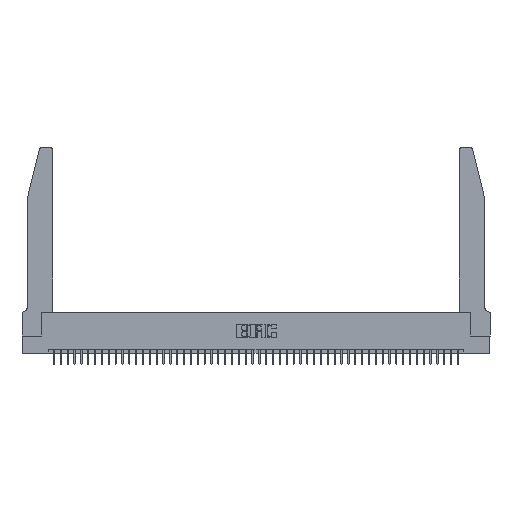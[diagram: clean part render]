
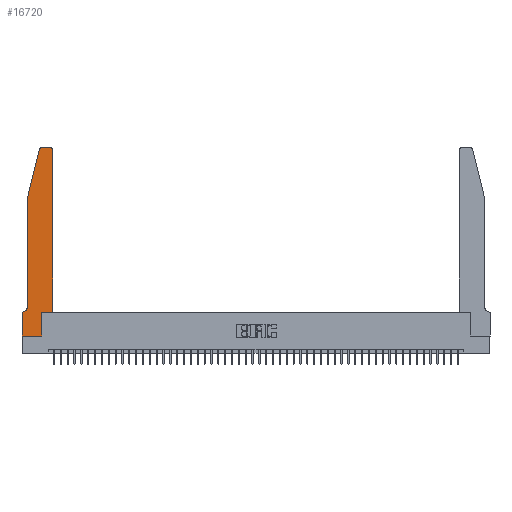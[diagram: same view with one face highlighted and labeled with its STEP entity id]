
A CAD part, top view. The second image highlights one B-rep face of the part: STEP entity #16720.
In plain terms, the highlighted planar face has unit normal (0, 0, 1).
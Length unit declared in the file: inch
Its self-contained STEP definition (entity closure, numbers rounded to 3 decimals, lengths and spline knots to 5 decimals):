
#959 = VERTEX_POINT ( 'NONE', #40195 ) ;
#1164 = DIRECTION ( 'NONE',  ( 0., -1., 0. ) ) ;
#1457 = VERTEX_POINT ( 'NONE', #7270 ) ;
#4528 = DIRECTION ( 'NONE',  ( 0., 0., 1. ) ) ;
#5020 = LINE ( 'NONE', #13585, #28966 ) ;
#5047 = VECTOR ( 'NONE', #10847, 39.37008 ) ;
#5134 = DIRECTION ( 'NONE',  ( 0., -1., 0. ) ) ;
#5814 = CARTESIAN_POINT ( 'NONE',  ( 0.4505, 0.35, 0.37 ) ) ;
#6054 = VERTEX_POINT ( 'NONE', #40809 ) ;
#6820 = CIRCLE ( 'NONE', #10229, 0.03 ) ;
#7005 = CARTESIAN_POINT ( 'NONE',  ( 0.4205, 2.72, 0.37 ) ) ;
#7157 = CARTESIAN_POINT ( 'NONE',  ( 0.0755, 2., 0.37 ) ) ;
#7270 = CARTESIAN_POINT ( 'NONE',  ( 0., 0.35, 0.37 ) ) ;
#7607 = CARTESIAN_POINT ( 'NONE',  ( 0.4205, 2.75, 0.37 ) ) ;
#8692 = CARTESIAN_POINT ( 'NONE',  ( 0.0755, 0.42, 0.37 ) ) ;
#9136 = EDGE_CURVE ( 'NONE', #26311, #43117, #32118, .T. ) ;
#9185 = VERTEX_POINT ( 'NONE', #48467 ) ;
#9391 = CARTESIAN_POINT ( 'NONE',  ( 0.4505, 2.72, 0.37 ) ) ;
#10101 = ORIENTED_EDGE ( 'NONE', *, *, #21083, .T. ) ;
#10229 = AXIS2_PLACEMENT_3D ( 'NONE', #7005, #22536, #26686 ) ;
#10551 = CARTESIAN_POINT ( 'NONE',  ( 0.2865, 0., 0.37 ) ) ;
#10623 = DIRECTION ( 'NONE',  ( 1., 0., 0. ) ) ;
#10847 = DIRECTION ( 'NONE',  ( -0.239, -0.971, 0. ) ) ;
#11303 = VERTEX_POINT ( 'NONE', #33861 ) ;
#11826 = VECTOR ( 'NONE', #21727, 39.37008 ) ;
#12398 = VECTOR ( 'NONE', #1164, 39.37008 ) ;
#12440 = DIRECTION ( 'NONE',  ( -1., 0., 0. ) ) ;
#12836 = ORIENTED_EDGE ( 'NONE', *, *, #31650, .T. ) ;
#13585 = CARTESIAN_POINT ( 'NONE',  ( 0.0755, 0.35, 0.37 ) ) ;
#13939 = CARTESIAN_POINT ( 'NONE',  ( 0., 0., 0.37 ) ) ;
#14050 = EDGE_CURVE ( 'NONE', #9185, #19016, #43178, .T. ) ;
#14434 = CARTESIAN_POINT ( 'NONE',  ( 0.4505, 0.35, 0.37 ) ) ;
#15198 = LINE ( 'NONE', #7157, #5047 ) ;
#15642 = DIRECTION ( 'NONE',  ( 1., 0., 0. ) ) ;
#15682 = VERTEX_POINT ( 'NONE', #44087 ) ;
#15969 = VERTEX_POINT ( 'NONE', #7607 ) ;
#16199 = PLANE ( 'NONE',  #27965 ) ;
#16534 = LINE ( 'NONE', #14434, #28512 ) ;
#16720 = ADVANCED_FACE ( 'NONE', ( #18972 ), #16199, .T. ) ;
#17407 = DIRECTION ( 'NONE',  ( -1., 0., 0. ) ) ;
#18972 = FACE_OUTER_BOUND ( 'NONE', #23552, .T. ) ;
#19016 = VERTEX_POINT ( 'NONE', #8692 ) ;
#19286 = ORIENTED_EDGE ( 'NONE', *, *, #9136, .T. ) ;
#19320 = ORIENTED_EDGE ( 'NONE', *, *, #38572, .T. ) ;
#21083 = EDGE_CURVE ( 'NONE', #41667, #15969, #6820, .T. ) ;
#21625 = VECTOR ( 'NONE', #39543, 39.37008 ) ;
#21727 = DIRECTION ( 'NONE',  ( 0., 1., 0. ) ) ;
#22536 = DIRECTION ( 'NONE',  ( 0., 0., 1. ) ) ;
#23552 = EDGE_LOOP ( 'NONE', ( #32612, #43770, #19320, #33153, #12836, #25225, #35252, #43160, #19286, #33865, #46588, #10101 ) ) ;
#24558 = CIRCLE ( 'NONE', #39953, 0.07 ) ;
#25225 = ORIENTED_EDGE ( 'NONE', *, *, #26791, .T. ) ;
#25535 = LINE ( 'NONE', #36167, #12398 ) ;
#26311 = VERTEX_POINT ( 'NONE', #10551 ) ;
#26686 = DIRECTION ( 'NONE',  ( 1., 0., 0. ) ) ;
#26791 = EDGE_CURVE ( 'NONE', #15682, #1457, #5020, .T. ) ;
#27951 = CARTESIAN_POINT ( 'NONE',  ( 0.0055, 0.42, 0.37 ) ) ;
#27965 = AXIS2_PLACEMENT_3D ( 'NONE', #38762, #4528, #35206 ) ;
#28012 = CARTESIAN_POINT ( 'NONE',  ( 0.0755, 2., 0.37 ) ) ;
#28512 = VECTOR ( 'NONE', #48211, 39.37008 ) ;
#28824 = LINE ( 'NONE', #5814, #21625 ) ;
#28966 = VECTOR ( 'NONE', #17407, 39.37008 ) ;
#30964 = CARTESIAN_POINT ( 'NONE',  ( 0.284, 2.72, 0.37 ) ) ;
#31107 = EDGE_CURVE ( 'NONE', #43117, #45739, #28824, .T. ) ;
#31618 = AXIS2_PLACEMENT_3D ( 'NONE', #30964, #35125, #15642 ) ;
#31650 = EDGE_CURVE ( 'NONE', #19016, #15682, #24558, .T. ) ;
#32118 = LINE ( 'NONE', #48303, #11826 ) ;
#32612 = ORIENTED_EDGE ( 'NONE', *, *, #36118, .T. ) ;
#32786 = EDGE_CURVE ( 'NONE', #11303, #6054, #47740, .T. ) ;
#33040 = LINE ( 'NONE', #34683, #37836 ) ;
#33153 = ORIENTED_EDGE ( 'NONE', *, *, #14050, .T. ) ;
#33861 = CARTESIAN_POINT ( 'NONE',  ( 0.284, 2.75, 0.37 ) ) ;
#33865 = ORIENTED_EDGE ( 'NONE', *, *, #31107, .T. ) ;
#34193 = DIRECTION ( 'NONE',  ( -1., 0., 0. ) ) ;
#34683 = CARTESIAN_POINT ( 'NONE',  ( 0.2605, 2.75, 0.37 ) ) ;
#35125 = DIRECTION ( 'NONE',  ( 0., 0., 1. ) ) ;
#35136 = VECTOR ( 'NONE', #10623, 39.37008 ) ;
#35206 = DIRECTION ( 'NONE',  ( 1., 0., 0. ) ) ;
#35252 = ORIENTED_EDGE ( 'NONE', *, *, #46805, .T. ) ;
#36118 = EDGE_CURVE ( 'NONE', #15969, #11303, #33040, .T. ) ;
#36167 = CARTESIAN_POINT ( 'NONE',  ( 0., 0., 0.37 ) ) ;
#37373 = EDGE_CURVE ( 'NONE', #45739, #41667, #16534, .T. ) ;
#37836 = VECTOR ( 'NONE', #34193, 39.37008 ) ;
#38572 = EDGE_CURVE ( 'NONE', #6054, #9185, #15198, .T. ) ;
#38762 = CARTESIAN_POINT ( 'NONE',  ( 0., 0.35, 0.37 ) ) ;
#39543 = DIRECTION ( 'NONE',  ( 1., 0., 0. ) ) ;
#39953 = AXIS2_PLACEMENT_3D ( 'NONE', #27951, #42670, #12440 ) ;
#40195 = CARTESIAN_POINT ( 'NONE',  ( 0., 0., 0.37 ) ) ;
#40809 = CARTESIAN_POINT ( 'NONE',  ( 0.25487, 2.72718, 0.37 ) ) ;
#41667 = VERTEX_POINT ( 'NONE', #9391 ) ;
#42670 = DIRECTION ( 'NONE',  ( 0., 0., -1. ) ) ;
#43117 = VERTEX_POINT ( 'NONE', #47130 ) ;
#43160 = ORIENTED_EDGE ( 'NONE', *, *, #45815, .T. ) ;
#43178 = LINE ( 'NONE', #28012, #46742 ) ;
#43770 = ORIENTED_EDGE ( 'NONE', *, *, #32786, .T. ) ;
#44087 = CARTESIAN_POINT ( 'NONE',  ( 0.0055, 0.35, 0.37 ) ) ;
#45356 = LINE ( 'NONE', #13939, #35136 ) ;
#45739 = VERTEX_POINT ( 'NONE', #48030 ) ;
#45815 = EDGE_CURVE ( 'NONE', #959, #26311, #45356, .T. ) ;
#46588 = ORIENTED_EDGE ( 'NONE', *, *, #37373, .T. ) ;
#46742 = VECTOR ( 'NONE', #5134, 39.37008 ) ;
#46805 = EDGE_CURVE ( 'NONE', #1457, #959, #25535, .T. ) ;
#47130 = CARTESIAN_POINT ( 'NONE',  ( 0.2865, 0.35, 0.37 ) ) ;
#47740 = CIRCLE ( 'NONE', #31618, 0.03 ) ;
#48030 = CARTESIAN_POINT ( 'NONE',  ( 0.4505, 0.35, 0.37 ) ) ;
#48211 = DIRECTION ( 'NONE',  ( 0., 1., 0. ) ) ;
#48303 = CARTESIAN_POINT ( 'NONE',  ( 0.2865, 0.35, 0.37 ) ) ;
#48467 = CARTESIAN_POINT ( 'NONE',  ( 0.0755, 2., 0.37 ) ) ;
